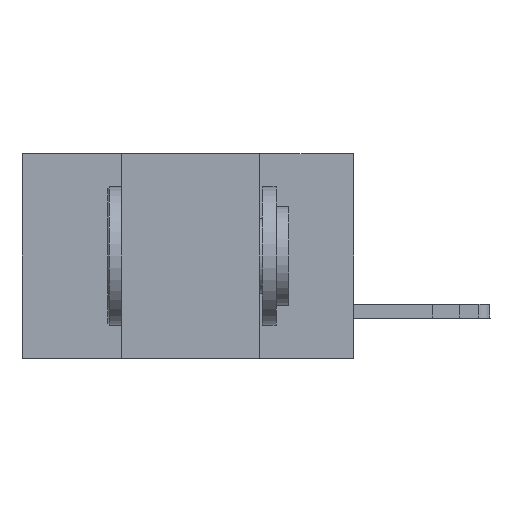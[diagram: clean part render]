
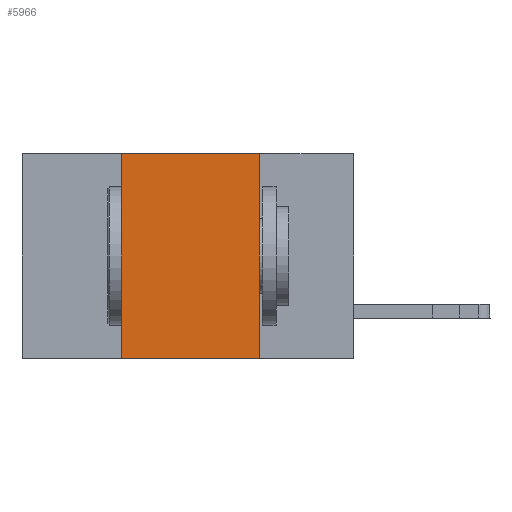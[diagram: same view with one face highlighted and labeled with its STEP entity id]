
A CAD part, left-side view. The second image highlights one B-rep face of the part: STEP entity #5966.
In plain terms, the highlighted planar face has unit normal (-1, 0, 0).
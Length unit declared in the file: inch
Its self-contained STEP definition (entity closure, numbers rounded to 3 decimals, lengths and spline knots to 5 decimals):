
#430 = VECTOR ( 'NONE', #4383, 39.37008 ) ;
#886 = CARTESIAN_POINT ( 'NONE',  ( 0., 0.6, -0.37 ) ) ;
#954 = CARTESIAN_POINT ( 'NONE',  ( 0., 0.42, 0. ) ) ;
#1867 = CARTESIAN_POINT ( 'NONE',  ( 0., 0.17, -0.37 ) ) ;
#4383 = DIRECTION ( 'NONE',  ( 0., -1., 0. ) ) ;
#4558 = LINE ( 'NONE', #26343, #30890 ) ;
#4857 = FACE_OUTER_BOUND ( 'NONE', #21675, .T. ) ;
#5966 = ADVANCED_FACE ( 'NONE', ( #4857 ), #12394, .F. ) ;
#9355 = LINE ( 'NONE', #23823, #28948 ) ;
#12394 = PLANE ( 'NONE',  #21621 ) ;
#12741 = VERTEX_POINT ( 'NONE', #1867 ) ;
#14951 = DIRECTION ( 'NONE',  ( 0., 0., -1. ) ) ;
#16510 = ORIENTED_EDGE ( 'NONE', *, *, #24587, .F. ) ;
#18396 = EDGE_CURVE ( 'NONE', #26194, #32758, #20743, .T. ) ;
#19231 = LINE ( 'NONE', #886, #31238 ) ;
#19778 = ORIENTED_EDGE ( 'NONE', *, *, #23314, .F. ) ;
#20133 = CARTESIAN_POINT ( 'NONE',  ( 0., 0.17, 0. ) ) ;
#20743 = LINE ( 'NONE', #32334, #430 ) ;
#21621 = AXIS2_PLACEMENT_3D ( 'NONE', #22574, #30260, #14951 ) ;
#21675 = EDGE_LOOP ( 'NONE', ( #19778, #31712, #16510, #25972 ) ) ;
#22574 = CARTESIAN_POINT ( 'NONE',  ( 0., 0.6, 0. ) ) ;
#23314 = EDGE_CURVE ( 'NONE', #32758, #12741, #9355, .T. ) ;
#23823 = CARTESIAN_POINT ( 'NONE',  ( 0., 0.17, 0. ) ) ;
#23982 = CARTESIAN_POINT ( 'NONE',  ( 0., 0.42, -0.37 ) ) ;
#24587 = EDGE_CURVE ( 'NONE', #28210, #26194, #4558, .T. ) ;
#25238 = EDGE_CURVE ( 'NONE', #28210, #12741, #19231, .T. ) ;
#25972 = ORIENTED_EDGE ( 'NONE', *, *, #25238, .T. ) ;
#26194 = VERTEX_POINT ( 'NONE', #954 ) ;
#26343 = CARTESIAN_POINT ( 'NONE',  ( 0., 0.42, 0. ) ) ;
#26403 = DIRECTION ( 'NONE',  ( 0., 0., -1. ) ) ;
#28210 = VERTEX_POINT ( 'NONE', #23982 ) ;
#28906 = DIRECTION ( 'NONE',  ( 0., 0., 1. ) ) ;
#28948 = VECTOR ( 'NONE', #26403, 39.37008 ) ;
#28974 = DIRECTION ( 'NONE',  ( 0., -1., 0. ) ) ;
#30260 = DIRECTION ( 'NONE',  ( 1., 0., 0. ) ) ;
#30890 = VECTOR ( 'NONE', #28906, 39.37008 ) ;
#31238 = VECTOR ( 'NONE', #28974, 39.37008 ) ;
#31712 = ORIENTED_EDGE ( 'NONE', *, *, #18396, .F. ) ;
#32334 = CARTESIAN_POINT ( 'NONE',  ( 0., 0.6, 0. ) ) ;
#32758 = VERTEX_POINT ( 'NONE', #20133 ) ;
